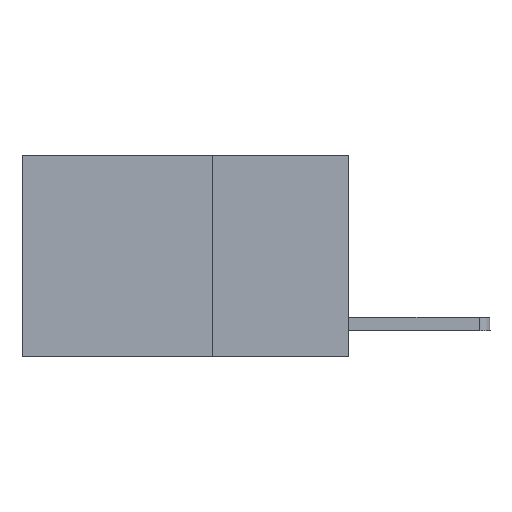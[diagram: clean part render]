
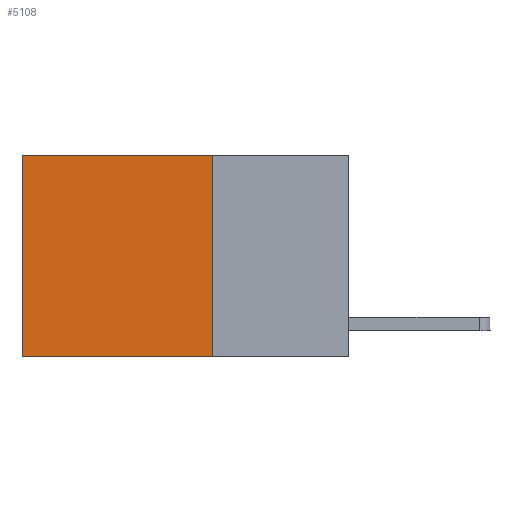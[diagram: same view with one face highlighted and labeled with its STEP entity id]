
A CAD part, left-side view. The second image highlights one B-rep face of the part: STEP entity #5108.
In plain terms, the highlighted planar face has unit normal (-1, 0, 0).
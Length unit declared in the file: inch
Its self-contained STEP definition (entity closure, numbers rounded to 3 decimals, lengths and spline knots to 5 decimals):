
#2 = EDGE_LOOP ( 'NONE', ( #6387, #4521, #2833, #1832 ) ) ;
#188 = CARTESIAN_POINT ( 'NONE',  ( 0.2625, 0.6, -0.37 ) ) ;
#293 = VERTEX_POINT ( 'NONE', #188 ) ;
#419 = VECTOR ( 'NONE', #7957, 39.37008 ) ;
#1083 = CARTESIAN_POINT ( 'NONE',  ( 0.2625, 0.25, 0. ) ) ;
#1127 = CARTESIAN_POINT ( 'NONE',  ( 0.2625, 0.25, 0. ) ) ;
#1605 = CARTESIAN_POINT ( 'NONE',  ( 0.2625, 0.25, 0. ) ) ;
#1772 = DIRECTION ( 'NONE',  ( 0., 0., -1. ) ) ;
#1832 = ORIENTED_EDGE ( 'NONE', *, *, #4278, .T. ) ;
#2315 = VECTOR ( 'NONE', #3254, 39.37008 ) ;
#2318 = LINE ( 'NONE', #6056, #419 ) ;
#2589 = CARTESIAN_POINT ( 'NONE',  ( 0.2625, 0.25, -0.37 ) ) ;
#2833 = ORIENTED_EDGE ( 'NONE', *, *, #6496, .F. ) ;
#2997 = CARTESIAN_POINT ( 'NONE',  ( 0.2625, 0.25, 0. ) ) ;
#3254 = DIRECTION ( 'NONE',  ( 0., 0., -1. ) ) ;
#3430 = FACE_OUTER_BOUND ( 'NONE', #2, .T. ) ;
#3833 = LINE ( 'NONE', #6354, #2315 ) ;
#4085 = DIRECTION ( 'NONE',  ( 1., 0., 0. ) ) ;
#4258 = EDGE_CURVE ( 'NONE', #4476, #293, #2318, .T. ) ;
#4277 = DIRECTION ( 'NONE',  ( 0., 1., 0. ) ) ;
#4278 = EDGE_CURVE ( 'NONE', #4773, #5528, #4806, .T. ) ;
#4476 = VERTEX_POINT ( 'NONE', #2589 ) ;
#4521 = ORIENTED_EDGE ( 'NONE', *, *, #4258, .F. ) ;
#4689 = CARTESIAN_POINT ( 'NONE',  ( 0.2625, 0.6, 0. ) ) ;
#4773 = VERTEX_POINT ( 'NONE', #1127 ) ;
#4806 = LINE ( 'NONE', #2997, #7561 ) ;
#5108 = ADVANCED_FACE ( 'NONE', ( #3430 ), #7169, .F. ) ;
#5364 = EDGE_CURVE ( 'NONE', #5528, #293, #3833, .T. ) ;
#5528 = VERTEX_POINT ( 'NONE', #4689 ) ;
#6056 = CARTESIAN_POINT ( 'NONE',  ( 0.2625, 0.25, -0.37 ) ) ;
#6354 = CARTESIAN_POINT ( 'NONE',  ( 0.2625, 0.6, 0. ) ) ;
#6387 = ORIENTED_EDGE ( 'NONE', *, *, #5364, .T. ) ;
#6496 = EDGE_CURVE ( 'NONE', #4773, #4476, #7983, .T. ) ;
#6562 = DIRECTION ( 'NONE',  ( 0., 0., -1. ) ) ;
#6766 = AXIS2_PLACEMENT_3D ( 'NONE', #1605, #4085, #6562 ) ;
#7169 = PLANE ( 'NONE',  #6766 ) ;
#7561 = VECTOR ( 'NONE', #4277, 39.37008 ) ;
#7957 = DIRECTION ( 'NONE',  ( 0., 1., 0. ) ) ;
#7983 = LINE ( 'NONE', #1083, #8012 ) ;
#8012 = VECTOR ( 'NONE', #1772, 39.37008 ) ;
